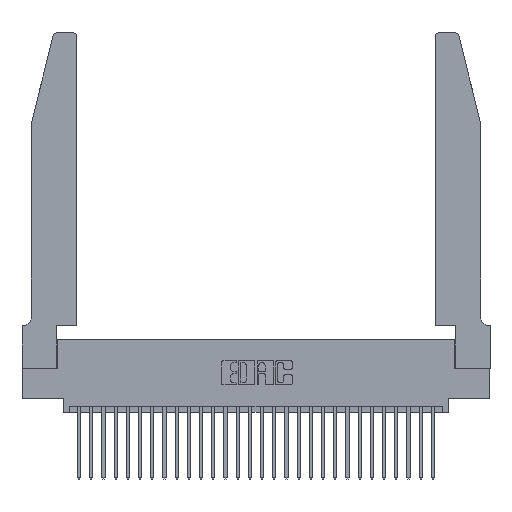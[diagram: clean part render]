
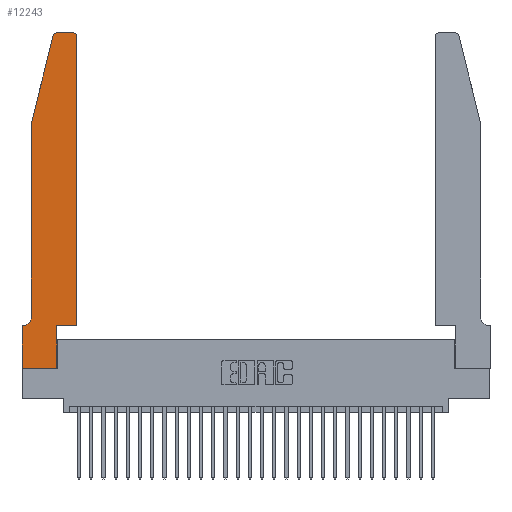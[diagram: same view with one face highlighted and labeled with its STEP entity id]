
A CAD part, top view. The second image highlights one B-rep face of the part: STEP entity #12243.
In plain terms, the highlighted planar face has unit normal (0, 0, 1).
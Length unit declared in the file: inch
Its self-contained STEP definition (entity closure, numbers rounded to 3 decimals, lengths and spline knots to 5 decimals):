
#197 = EDGE_LOOP ( 'NONE', ( #26623, #29849, #27917, #26353, #12264, #12899, #28772, #15657, #29178, #21635, #6085, #3889 ) ) ;
#213 = FACE_OUTER_BOUND ( 'NONE', #197, .T. ) ;
#1131 = VERTEX_POINT ( 'NONE', #8932 ) ;
#1578 = CARTESIAN_POINT ( 'NONE',  ( 0.2605, 2.75, 0.37 ) ) ;
#2159 = AXIS2_PLACEMENT_3D ( 'NONE', #20049, #5864, #4453 ) ;
#2514 = LINE ( 'NONE', #14734, #18133 ) ;
#2770 = DIRECTION ( 'NONE',  ( 0., 1., 0. ) ) ;
#2941 = CIRCLE ( 'NONE', #28061, 0.03 ) ;
#2945 = LINE ( 'NONE', #1578, #5489 ) ;
#3215 = EDGE_CURVE ( 'NONE', #4975, #16108, #5796, .T. ) ;
#3502 = VECTOR ( 'NONE', #13028, 39.37008 ) ;
#3851 = EDGE_CURVE ( 'NONE', #16555, #1131, #2514, .T. ) ;
#3889 = ORIENTED_EDGE ( 'NONE', *, *, #3215, .T. ) ;
#4089 = VERTEX_POINT ( 'NONE', #27774 ) ;
#4306 = VERTEX_POINT ( 'NONE', #7037 ) ;
#4453 = DIRECTION ( 'NONE',  ( -1., 0., 0. ) ) ;
#4747 = EDGE_CURVE ( 'NONE', #1131, #4089, #27938, .T. ) ;
#4975 = VERTEX_POINT ( 'NONE', #22988 ) ;
#5264 = VECTOR ( 'NONE', #9356, 39.37008 ) ;
#5489 = VECTOR ( 'NONE', #28283, 39.37008 ) ;
#5750 = EDGE_CURVE ( 'NONE', #18543, #17681, #26771, .T. ) ;
#5796 = CIRCLE ( 'NONE', #22443, 0.03 ) ;
#5864 = DIRECTION ( 'NONE',  ( 0., 0., -1. ) ) ;
#6085 = ORIENTED_EDGE ( 'NONE', *, *, #17478, .T. ) ;
#7003 = CARTESIAN_POINT ( 'NONE',  ( 0.0755, 2., 0.37 ) ) ;
#7037 = CARTESIAN_POINT ( 'NONE',  ( 0.2865, 0.35, 0.37 ) ) ;
#8932 = CARTESIAN_POINT ( 'NONE',  ( 0., 0.35, 0.37 ) ) ;
#8952 = DIRECTION ( 'NONE',  ( 1., 0., 0. ) ) ;
#9050 = CARTESIAN_POINT ( 'NONE',  ( 0.4505, 0.35, 0.37 ) ) ;
#9356 = DIRECTION ( 'NONE',  ( 1., 0., 0. ) ) ;
#10002 = VECTOR ( 'NONE', #21854, 39.37008 ) ;
#10023 = CIRCLE ( 'NONE', #2159, 0.07 ) ;
#10080 = VERTEX_POINT ( 'NONE', #21910 ) ;
#10305 = CARTESIAN_POINT ( 'NONE',  ( 0.0755, 2., 0.37 ) ) ;
#10311 = DIRECTION ( 'NONE',  ( 1., 0., 0. ) ) ;
#12243 = ADVANCED_FACE ( 'NONE', ( #213 ), #19000, .T. ) ;
#12264 = ORIENTED_EDGE ( 'NONE', *, *, #13722, .T. ) ;
#12300 = LINE ( 'NONE', #9050, #18064 ) ;
#12506 = DIRECTION ( 'NONE',  ( 0., 0., 1. ) ) ;
#12899 = ORIENTED_EDGE ( 'NONE', *, *, #3851, .T. ) ;
#13028 = DIRECTION ( 'NONE',  ( 0., -1., 0. ) ) ;
#13677 = EDGE_CURVE ( 'NONE', #4089, #10080, #21930, .T. ) ;
#13722 = EDGE_CURVE ( 'NONE', #17681, #16555, #10023, .T. ) ;
#13949 = DIRECTION ( 'NONE',  ( 0., 1., 0. ) ) ;
#14404 = CARTESIAN_POINT ( 'NONE',  ( 0.2865, 0.35, 0.37 ) ) ;
#14734 = CARTESIAN_POINT ( 'NONE',  ( 0.0755, 0.35, 0.37 ) ) ;
#15532 = CARTESIAN_POINT ( 'NONE',  ( 0.4505, 0.35, 0.37 ) ) ;
#15657 = ORIENTED_EDGE ( 'NONE', *, *, #13677, .T. ) ;
#15828 = CARTESIAN_POINT ( 'NONE',  ( 0.4505, 0.35, 0.37 ) ) ;
#16108 = VERTEX_POINT ( 'NONE', #19724 ) ;
#16307 = EDGE_CURVE ( 'NONE', #16108, #24815, #2945, .T. ) ;
#16504 = CARTESIAN_POINT ( 'NONE',  ( 0., 0., 0.37 ) ) ;
#16555 = VERTEX_POINT ( 'NONE', #29157 ) ;
#17072 = CARTESIAN_POINT ( 'NONE',  ( 0.25487, 2.72718, 0.37 ) ) ;
#17307 = CARTESIAN_POINT ( 'NONE',  ( 0.0755, 2., 0.37 ) ) ;
#17433 = DIRECTION ( 'NONE',  ( 0., 0., 1. ) ) ;
#17478 = EDGE_CURVE ( 'NONE', #29513, #4975, #12300, .T. ) ;
#17584 = LINE ( 'NONE', #17307, #10002 ) ;
#17681 = VERTEX_POINT ( 'NONE', #22831 ) ;
#18064 = VECTOR ( 'NONE', #13949, 39.37008 ) ;
#18071 = VECTOR ( 'NONE', #2770, 39.37008 ) ;
#18133 = VECTOR ( 'NONE', #21856, 39.37008 ) ;
#18543 = VERTEX_POINT ( 'NONE', #7003 ) ;
#18882 = AXIS2_PLACEMENT_3D ( 'NONE', #21618, #21914, #10311 ) ;
#19000 = PLANE ( 'NONE',  #18882 ) ;
#19519 = LINE ( 'NONE', #14404, #18071 ) ;
#19553 = VECTOR ( 'NONE', #28209, 39.37008 ) ;
#19702 = EDGE_CURVE ( 'NONE', #27640, #18543, #17584, .T. ) ;
#19724 = CARTESIAN_POINT ( 'NONE',  ( 0.4205, 2.75, 0.37 ) ) ;
#20006 = VECTOR ( 'NONE', #8952, 39.37008 ) ;
#20049 = CARTESIAN_POINT ( 'NONE',  ( 0.0055, 0.42, 0.37 ) ) ;
#20888 = CARTESIAN_POINT ( 'NONE',  ( 0., 0., 0.37 ) ) ;
#21618 = CARTESIAN_POINT ( 'NONE',  ( 0., 0.35, 0.37 ) ) ;
#21635 = ORIENTED_EDGE ( 'NONE', *, *, #29460, .T. ) ;
#21794 = LINE ( 'NONE', #15532, #20006 ) ;
#21854 = DIRECTION ( 'NONE',  ( -0.239, -0.971, 0. ) ) ;
#21856 = DIRECTION ( 'NONE',  ( -1., 0., 0. ) ) ;
#21910 = CARTESIAN_POINT ( 'NONE',  ( 0.2865, 0., 0.37 ) ) ;
#21914 = DIRECTION ( 'NONE',  ( 0., 0., 1. ) ) ;
#21930 = LINE ( 'NONE', #20888, #5264 ) ;
#22090 = DIRECTION ( 'NONE',  ( 1., 0., 0. ) ) ;
#22443 = AXIS2_PLACEMENT_3D ( 'NONE', #28207, #12506, #28699 ) ;
#22831 = CARTESIAN_POINT ( 'NONE',  ( 0.0755, 0.42, 0.37 ) ) ;
#22988 = CARTESIAN_POINT ( 'NONE',  ( 0.4505, 2.72, 0.37 ) ) ;
#24815 = VERTEX_POINT ( 'NONE', #25028 ) ;
#25028 = CARTESIAN_POINT ( 'NONE',  ( 0.284, 2.75, 0.37 ) ) ;
#25729 = EDGE_CURVE ( 'NONE', #10080, #4306, #19519, .T. ) ;
#26353 = ORIENTED_EDGE ( 'NONE', *, *, #5750, .T. ) ;
#26608 = CARTESIAN_POINT ( 'NONE',  ( 0.284, 2.72, 0.37 ) ) ;
#26623 = ORIENTED_EDGE ( 'NONE', *, *, #16307, .T. ) ;
#26771 = LINE ( 'NONE', #10305, #3502 ) ;
#27640 = VERTEX_POINT ( 'NONE', #17072 ) ;
#27774 = CARTESIAN_POINT ( 'NONE',  ( 0., 0., 0.37 ) ) ;
#27917 = ORIENTED_EDGE ( 'NONE', *, *, #19702, .T. ) ;
#27938 = LINE ( 'NONE', #16504, #19553 ) ;
#28061 = AXIS2_PLACEMENT_3D ( 'NONE', #26608, #17433, #22090 ) ;
#28207 = CARTESIAN_POINT ( 'NONE',  ( 0.4205, 2.72, 0.37 ) ) ;
#28209 = DIRECTION ( 'NONE',  ( 0., -1., 0. ) ) ;
#28283 = DIRECTION ( 'NONE',  ( -1., 0., 0. ) ) ;
#28699 = DIRECTION ( 'NONE',  ( 1., 0., 0. ) ) ;
#28772 = ORIENTED_EDGE ( 'NONE', *, *, #4747, .T. ) ;
#29157 = CARTESIAN_POINT ( 'NONE',  ( 0.0055, 0.35, 0.37 ) ) ;
#29178 = ORIENTED_EDGE ( 'NONE', *, *, #25729, .T. ) ;
#29270 = EDGE_CURVE ( 'NONE', #24815, #27640, #2941, .T. ) ;
#29460 = EDGE_CURVE ( 'NONE', #4306, #29513, #21794, .T. ) ;
#29513 = VERTEX_POINT ( 'NONE', #15828 ) ;
#29849 = ORIENTED_EDGE ( 'NONE', *, *, #29270, .T. ) ;
